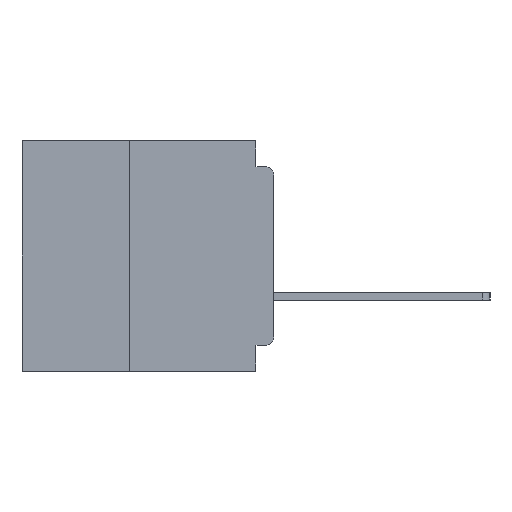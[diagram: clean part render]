
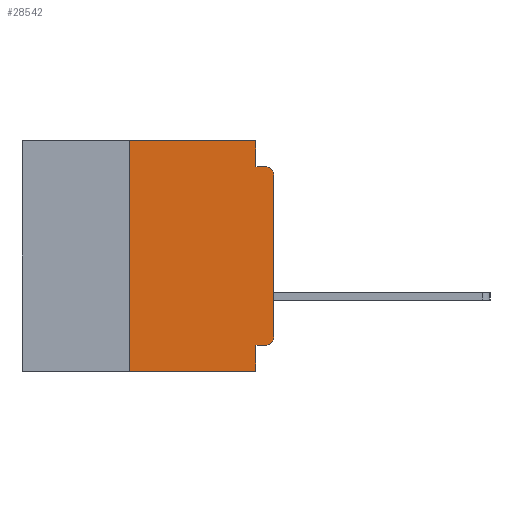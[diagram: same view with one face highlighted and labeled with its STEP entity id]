
A CAD part, left-side view. The second image highlights one B-rep face of the part: STEP entity #28542.
In plain terms, the highlighted planar face has unit normal (-1, 0, 0).
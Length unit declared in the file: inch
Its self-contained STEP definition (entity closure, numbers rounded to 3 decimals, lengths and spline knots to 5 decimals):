
#182 = LINE ( 'NONE', #10817, #21878 ) ;
#1575 = VECTOR ( 'NONE', #5856, 39.37008 ) ;
#1916 = CARTESIAN_POINT ( 'NONE',  ( 0., 0.015, -0.06 ) ) ;
#2757 = CARTESIAN_POINT ( 'NONE',  ( 0., 0.25, -0.4 ) ) ;
#2979 = VERTEX_POINT ( 'NONE', #17053 ) ;
#3552 = CIRCLE ( 'NONE', #32332, 0.015 ) ;
#3719 = ORIENTED_EDGE ( 'NONE', *, *, #18239, .T. ) ;
#3930 = DIRECTION ( 'NONE',  ( -1., 0., 0. ) ) ;
#4756 = EDGE_CURVE ( 'NONE', #13238, #2979, #35597, .T. ) ;
#4892 = DIRECTION ( 'NONE',  ( 0., 0., -1. ) ) ;
#5025 = LINE ( 'NONE', #33807, #19742 ) ;
#5283 = VECTOR ( 'NONE', #15632, 39.37008 ) ;
#5313 = ORIENTED_EDGE ( 'NONE', *, *, #34265, .T. ) ;
#5856 = DIRECTION ( 'NONE',  ( 0., 0., 1. ) ) ;
#7087 = CARTESIAN_POINT ( 'NONE',  ( 0., 0.031, -0.045 ) ) ;
#7182 = VERTEX_POINT ( 'NONE', #19746 ) ;
#7736 = CARTESIAN_POINT ( 'NONE',  ( 0., 0., -0.34 ) ) ;
#7806 = VERTEX_POINT ( 'NONE', #9014 ) ;
#7808 = ORIENTED_EDGE ( 'NONE', *, *, #11658, .F. ) ;
#8243 = CARTESIAN_POINT ( 'NONE',  ( 0., 0., -0.06 ) ) ;
#8329 = CARTESIAN_POINT ( 'NONE',  ( 0., 0., 0. ) ) ;
#8907 = VECTOR ( 'NONE', #11374, 39.37008 ) ;
#8923 = AXIS2_PLACEMENT_3D ( 'NONE', #1916, #22545, #4892 ) ;
#9014 = CARTESIAN_POINT ( 'NONE',  ( 0., 0.25, 0. ) ) ;
#9173 = ORIENTED_EDGE ( 'NONE', *, *, #15512, .F. ) ;
#9236 = EDGE_CURVE ( 'NONE', #7182, #36509, #3552, .T. ) ;
#9545 = VERTEX_POINT ( 'NONE', #8243 ) ;
#10020 = DIRECTION ( 'NONE',  ( 1., 0., 0. ) ) ;
#10817 = CARTESIAN_POINT ( 'NONE',  ( 0., 0.437, 0. ) ) ;
#11286 = DIRECTION ( 'NONE',  ( 0., 0., 1. ) ) ;
#11374 = DIRECTION ( 'NONE',  ( 0., -1., 0. ) ) ;
#11658 = EDGE_CURVE ( 'NONE', #22140, #36967, #26978, .T. ) ;
#11719 = EDGE_CURVE ( 'NONE', #33232, #7806, #31018, .T. ) ;
#11720 = CARTESIAN_POINT ( 'NONE',  ( 0., 0.25, -0.4 ) ) ;
#12183 = ORIENTED_EDGE ( 'NONE', *, *, #9236, .T. ) ;
#13238 = VERTEX_POINT ( 'NONE', #36810 ) ;
#13701 = FACE_OUTER_BOUND ( 'NONE', #34734, .T. ) ;
#14901 = ORIENTED_EDGE ( 'NONE', *, *, #20347, .T. ) ;
#15150 = EDGE_CURVE ( 'NONE', #7182, #13238, #20947, .T. ) ;
#15512 = EDGE_CURVE ( 'NONE', #36967, #25335, #16709, .T. ) ;
#15632 = DIRECTION ( 'NONE',  ( 0., 1., 0. ) ) ;
#15920 = CARTESIAN_POINT ( 'NONE',  ( 0., 0.437, 0. ) ) ;
#16709 = LINE ( 'NONE', #23297, #8907 ) ;
#16798 = CARTESIAN_POINT ( 'NONE',  ( 0., 0.031, 0. ) ) ;
#17053 = CARTESIAN_POINT ( 'NONE',  ( 0., 0.031, -0.4 ) ) ;
#17253 = DIRECTION ( 'NONE',  ( 0., 0., -1. ) ) ;
#18239 = EDGE_CURVE ( 'NONE', #33232, #2979, #5025, .T. ) ;
#18953 = PLANE ( 'NONE',  #26128 ) ;
#19597 = DIRECTION ( 'NONE',  ( 0., -1., 0. ) ) ;
#19742 = VECTOR ( 'NONE', #25027, 39.37008 ) ;
#19746 = CARTESIAN_POINT ( 'NONE',  ( 0., 0.015, -0.355 ) ) ;
#19790 = CARTESIAN_POINT ( 'NONE',  ( 0., 0.031, -0.4 ) ) ;
#20229 = CARTESIAN_POINT ( 'NONE',  ( 0., 0.015, -0.045 ) ) ;
#20347 = EDGE_CURVE ( 'NONE', #36509, #9545, #35465, .T. ) ;
#20947 = LINE ( 'NONE', #33273, #5283 ) ;
#21575 = CARTESIAN_POINT ( 'NONE',  ( 0., 0.015, -0.34 ) ) ;
#21878 = VECTOR ( 'NONE', #19597, 39.37008 ) ;
#21918 = DIRECTION ( 'NONE',  ( 0., 0., -1. ) ) ;
#22140 = VERTEX_POINT ( 'NONE', #16798 ) ;
#22545 = DIRECTION ( 'NONE',  ( -1., 0., 0. ) ) ;
#23055 = ORIENTED_EDGE ( 'NONE', *, *, #4756, .F. ) ;
#23130 = CARTESIAN_POINT ( 'NONE',  ( 0., 0.031, 0. ) ) ;
#23297 = CARTESIAN_POINT ( 'NONE',  ( 0., 0., -0.045 ) ) ;
#24570 = DIRECTION ( 'NONE',  ( 0., 0., -1. ) ) ;
#25027 = DIRECTION ( 'NONE',  ( 0., -1., 0. ) ) ;
#25081 = CIRCLE ( 'NONE', #8923, 0.015 ) ;
#25335 = VERTEX_POINT ( 'NONE', #20229 ) ;
#26128 = AXIS2_PLACEMENT_3D ( 'NONE', #15920, #10020, #21918 ) ;
#26978 = LINE ( 'NONE', #23130, #33772 ) ;
#27852 = VECTOR ( 'NONE', #31602, 39.37008 ) ;
#28542 = ADVANCED_FACE ( 'NONE', ( #13701 ), #18953, .F. ) ;
#31018 = LINE ( 'NONE', #11720, #1575 ) ;
#31602 = DIRECTION ( 'NONE',  ( 0., 0., -1. ) ) ;
#32332 = AXIS2_PLACEMENT_3D ( 'NONE', #21575, #3930, #24570 ) ;
#33232 = VERTEX_POINT ( 'NONE', #2757 ) ;
#33273 = CARTESIAN_POINT ( 'NONE',  ( 0., 0., -0.355 ) ) ;
#33714 = EDGE_CURVE ( 'NONE', #7806, #22140, #182, .T. ) ;
#33772 = VECTOR ( 'NONE', #17253, 39.37008 ) ;
#33807 = CARTESIAN_POINT ( 'NONE',  ( 0., 0.437, -0.4 ) ) ;
#34265 = EDGE_CURVE ( 'NONE', #9545, #25335, #25081, .T. ) ;
#34536 = VECTOR ( 'NONE', #11286, 39.37008 ) ;
#34734 = EDGE_LOOP ( 'NONE', ( #14901, #5313, #9173, #7808, #37430, #37087, #3719, #23055, #36073, #12183 ) ) ;
#35465 = LINE ( 'NONE', #8329, #34536 ) ;
#35597 = LINE ( 'NONE', #19790, #27852 ) ;
#36073 = ORIENTED_EDGE ( 'NONE', *, *, #15150, .F. ) ;
#36509 = VERTEX_POINT ( 'NONE', #7736 ) ;
#36810 = CARTESIAN_POINT ( 'NONE',  ( 0., 0.031, -0.355 ) ) ;
#36967 = VERTEX_POINT ( 'NONE', #7087 ) ;
#37087 = ORIENTED_EDGE ( 'NONE', *, *, #11719, .F. ) ;
#37430 = ORIENTED_EDGE ( 'NONE', *, *, #33714, .F. ) ;
